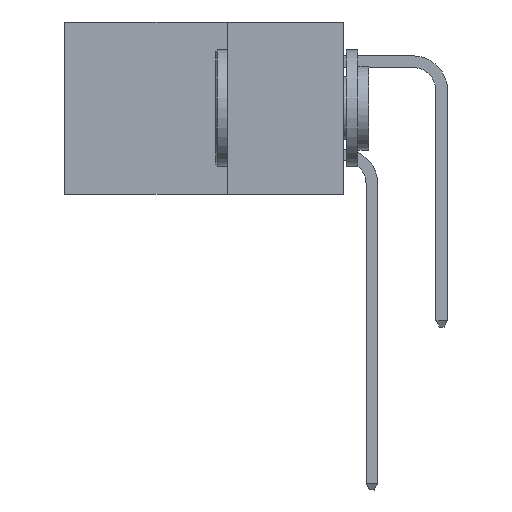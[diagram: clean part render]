
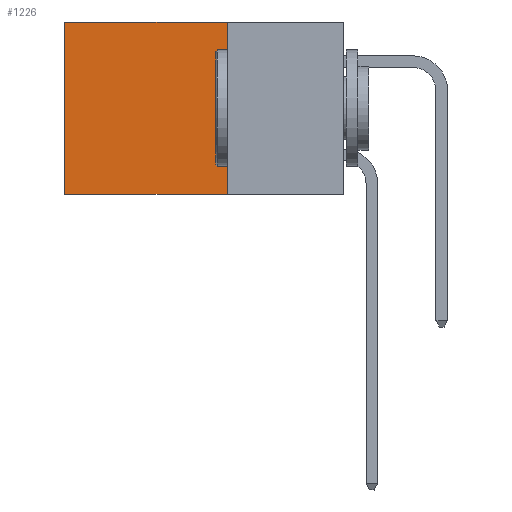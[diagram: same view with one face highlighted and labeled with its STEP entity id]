
A CAD part, left-side view. The second image highlights one B-rep face of the part: STEP entity #1226.
In plain terms, the highlighted planar face has unit normal (-1, 0, 0).
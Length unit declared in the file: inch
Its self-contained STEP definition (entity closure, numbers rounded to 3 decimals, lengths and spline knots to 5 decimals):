
#257 = DIRECTION ( 'NONE',  ( 0., 0., -1. ) ) ;
#465 = VERTEX_POINT ( 'NONE', #2519 ) ;
#623 = VERTEX_POINT ( 'NONE', #7817 ) ;
#1096 = CARTESIAN_POINT ( 'NONE',  ( 0.2615, 0.25, -0.37 ) ) ;
#1226 = ADVANCED_FACE ( 'NONE', ( #9302 ), #11264, .F. ) ;
#1535 = CARTESIAN_POINT ( 'NONE',  ( 0.2615, 0.25, 0. ) ) ;
#1717 = VERTEX_POINT ( 'NONE', #1535 ) ;
#1838 = VECTOR ( 'NONE', #12904, 39.37008 ) ;
#2102 = DIRECTION ( 'NONE',  ( 1., 0., 0. ) ) ;
#2194 = EDGE_CURVE ( 'NONE', #465, #10713, #5535, .T. ) ;
#2232 = CARTESIAN_POINT ( 'NONE',  ( 0.2615, 0.25, -0.37 ) ) ;
#2519 = CARTESIAN_POINT ( 'NONE',  ( 0.2615, 0.6, 0. ) ) ;
#2669 = LINE ( 'NONE', #4580, #1838 ) ;
#2983 = DIRECTION ( 'NONE',  ( 0., 1., 0. ) ) ;
#3106 = ORIENTED_EDGE ( 'NONE', *, *, #2194, .T. ) ;
#3274 = LINE ( 'NONE', #1096, #7569 ) ;
#4580 = CARTESIAN_POINT ( 'NONE',  ( 0.2615, 0.25, -0.37 ) ) ;
#5024 = LINE ( 'NONE', #7146, #9649 ) ;
#5535 = LINE ( 'NONE', #12557, #6892 ) ;
#5776 = ORIENTED_EDGE ( 'NONE', *, *, #8363, .F. ) ;
#6451 = ORIENTED_EDGE ( 'NONE', *, *, #11891, .F. ) ;
#6489 = DIRECTION ( 'NONE',  ( 0., 0., -1. ) ) ;
#6892 = VECTOR ( 'NONE', #6489, 39.37008 ) ;
#7146 = CARTESIAN_POINT ( 'NONE',  ( 0.2615, 0.25, 0. ) ) ;
#7312 = EDGE_CURVE ( 'NONE', #1717, #465, #5024, .T. ) ;
#7569 = VECTOR ( 'NONE', #8312, 39.37008 ) ;
#7700 = EDGE_LOOP ( 'NONE', ( #3106, #5776, #6451, #10617 ) ) ;
#7817 = CARTESIAN_POINT ( 'NONE',  ( 0.2615, 0.25, -0.37 ) ) ;
#8312 = DIRECTION ( 'NONE',  ( 0., 1., 0. ) ) ;
#8363 = EDGE_CURVE ( 'NONE', #623, #10713, #3274, .T. ) ;
#9302 = FACE_OUTER_BOUND ( 'NONE', #7700, .T. ) ;
#9649 = VECTOR ( 'NONE', #2983, 39.37008 ) ;
#10008 = AXIS2_PLACEMENT_3D ( 'NONE', #2232, #2102, #257 ) ;
#10617 = ORIENTED_EDGE ( 'NONE', *, *, #7312, .T. ) ;
#10713 = VERTEX_POINT ( 'NONE', #12098 ) ;
#11264 = PLANE ( 'NONE',  #10008 ) ;
#11891 = EDGE_CURVE ( 'NONE', #1717, #623, #2669, .T. ) ;
#12098 = CARTESIAN_POINT ( 'NONE',  ( 0.2615, 0.6, -0.37 ) ) ;
#12557 = CARTESIAN_POINT ( 'NONE',  ( 0.2615, 0.6, -0.37 ) ) ;
#12904 = DIRECTION ( 'NONE',  ( 0., 0., -1. ) ) ;
